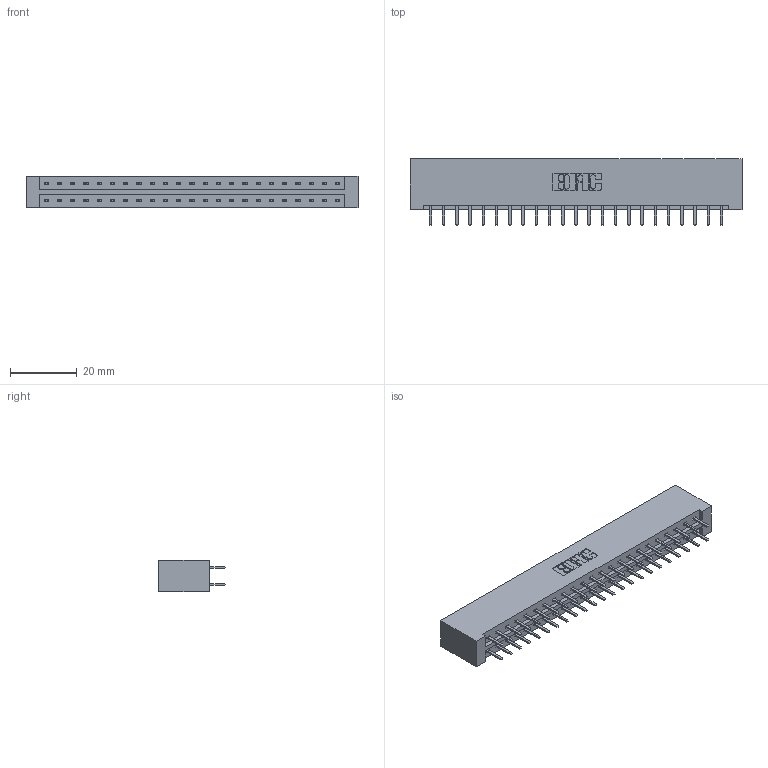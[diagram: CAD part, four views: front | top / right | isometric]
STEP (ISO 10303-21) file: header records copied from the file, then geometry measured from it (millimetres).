
FILE_DESCRIPTION (( 'STEP AP203' ), '1' );
FILE_NAME ('833-046-520-201.STEP', '2020-06-04T13:50:31', ( '' ), ( '' ), 'SwSTEP 2.0', 'SolidWorks 2020', '' );
FILE_SCHEMA (( 'CONFIG_CONTROL_DESIGN' ));
Length unit declared in the file: inch
Products named in the file (3): 833-046-520-201; 833 Part_Lugless; 345-292-001_345-293-120
Assembly tree (47 placements, depth 2):
  833-046-520-201
    833 Part_Lugless
    345-292-001_345-293-120  x46
Bounding box: 99.39 x 20.02 x 9.4 mm (x, y, z)
Volume: 10581.5 mm3; surface area: 12276.6 mm2
Topology: 47 solids, 47 shells, 2682 faces, 7785 edges, 5066 vertices
Faces by surface type: plane 1814, cylinder 868
Entity records: 17091 total; most frequent: CARTESIAN_POINT 2866, ORIENTED_EDGE 2790, DIRECTION 2463, EDGE_CURVE 1395, LINE 1271, VECTOR 1271, VERTEX_POINT 926, AXIS2_PLACEMENT_3D 596
